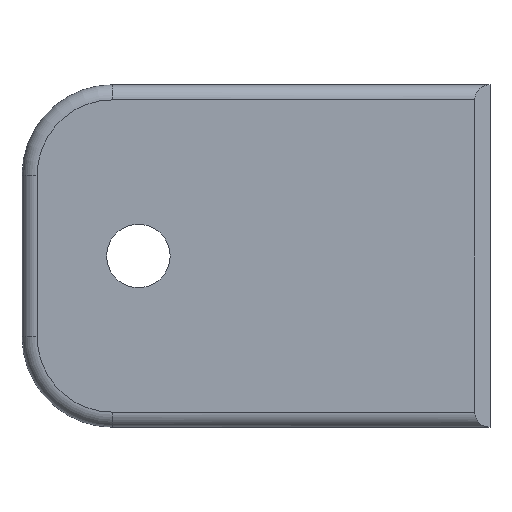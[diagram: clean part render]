
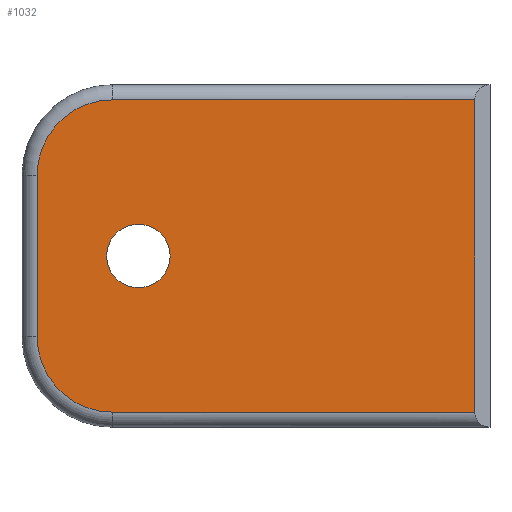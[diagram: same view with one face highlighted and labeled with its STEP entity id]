
A CAD part, front view. The second image highlights one B-rep face of the part: STEP entity #1032.
In plain terms, the highlighted planar face has unit normal (0, -1, 0).
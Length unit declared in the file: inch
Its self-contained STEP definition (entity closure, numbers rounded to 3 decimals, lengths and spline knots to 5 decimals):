
#24=PLANE('',#1161);
#77=LINE('',#1959,#152);
#80=LINE('',#1974,#155);
#82=LINE('',#1986,#157);
#83=LINE('',#1988,#158);
#152=VECTOR('',#1391,0.3937);
#155=VECTOR('',#1408,0.3937);
#157=VECTOR('',#1422,0.3937);
#158=VECTOR('',#1425,0.3937);
#232=FACE_BOUND('',#340,.T.);
#273=FACE_OUTER_BOUND('',#339,.T.);
#339=EDGE_LOOP('',(#840,#841,#842,#843,#844,#845));
#340=EDGE_LOOP('',(#846));
#364=CIRCLE('',#1077,0.105);
#394=CIRCLE('',#1152,0.25);
#398=CIRCLE('',#1158,0.25);
#410=VERTEX_POINT('',#1533);
#471=VERTEX_POINT('',#1956);
#472=VERTEX_POINT('',#1958);
#474=VERTEX_POINT('',#1964);
#476=VERTEX_POINT('',#1970);
#478=VERTEX_POINT('',#1976);
#480=VERTEX_POINT('',#1982);
#502=EDGE_CURVE('',#410,#410,#364,.T.);
#596=EDGE_CURVE('',#471,#472,#77,.T.);
#601=EDGE_CURVE('',#472,#474,#394,.T.);
#604=EDGE_CURVE('',#474,#476,#80,.T.);
#607=EDGE_CURVE('',#476,#478,#398,.T.);
#610=EDGE_CURVE('',#478,#480,#82,.T.);
#611=EDGE_CURVE('',#480,#471,#83,.T.);
#840=ORIENTED_EDGE('',*,*,#610,.F.);
#841=ORIENTED_EDGE('',*,*,#607,.F.);
#842=ORIENTED_EDGE('',*,*,#604,.F.);
#843=ORIENTED_EDGE('',*,*,#601,.F.);
#844=ORIENTED_EDGE('',*,*,#596,.F.);
#845=ORIENTED_EDGE('',*,*,#611,.F.);
#846=ORIENTED_EDGE('',*,*,#502,.T.);
#1032=ADVANCED_FACE('',(#273,#232),#24,.F.);
#1077=AXIS2_PLACEMENT_3D('',#1534,#1206,#1207);
#1152=AXIS2_PLACEMENT_3D('',#1968,#1401,#1402);
#1158=AXIS2_PLACEMENT_3D('',#1980,#1415,#1416);
#1161=AXIS2_PLACEMENT_3D('',#1987,#1423,#1424);
#1206=DIRECTION('center_axis',(0.,1.,0.));
#1207=DIRECTION('ref_axis',(-1.,0.,0.));
#1391=DIRECTION('',(-1.,0.,0.));
#1401=DIRECTION('center_axis',(0.,1.,0.));
#1402=DIRECTION('ref_axis',(-0.707,0.,-0.707));
#1408=DIRECTION('',(0.,0.,1.));
#1415=DIRECTION('center_axis',(0.,1.,0.));
#1416=DIRECTION('ref_axis',(-0.707,0.,0.707));
#1422=DIRECTION('',(1.,0.,0.));
#1423=DIRECTION('center_axis',(0.,1.,0.));
#1424=DIRECTION('ref_axis',(0.,0.,1.));
#1425=DIRECTION('',(0.,0.,-1.));
#1533=CARTESIAN_POINT('',(0.49,0.,-0.5665));
#1534=CARTESIAN_POINT('Origin',(0.385,0.,-0.5665));
#1956=CARTESIAN_POINT('',(1.498,0.,-1.083));
#1958=CARTESIAN_POINT('',(0.3,0.,-1.083));
#1959=CARTESIAN_POINT('',(1.161,0.,-1.083));
#1964=CARTESIAN_POINT('',(0.05,0.,-0.833));
#1968=CARTESIAN_POINT('Origin',(0.3,0.,-0.833));
#1970=CARTESIAN_POINT('',(0.05,0.,-0.3));
#1974=CARTESIAN_POINT('',(0.05,0.,-0.84975));
#1976=CARTESIAN_POINT('',(0.3,0.,-0.05));
#1980=CARTESIAN_POINT('Origin',(0.3,0.,-0.3));
#1982=CARTESIAN_POINT('',(1.498,0.,-0.05));
#1986=CARTESIAN_POINT('',(0.387,0.,-0.05));
#1987=CARTESIAN_POINT('Origin',(0.774,0.,-0.5665));
#1988=CARTESIAN_POINT('',(1.498,0.,-0.28325));
